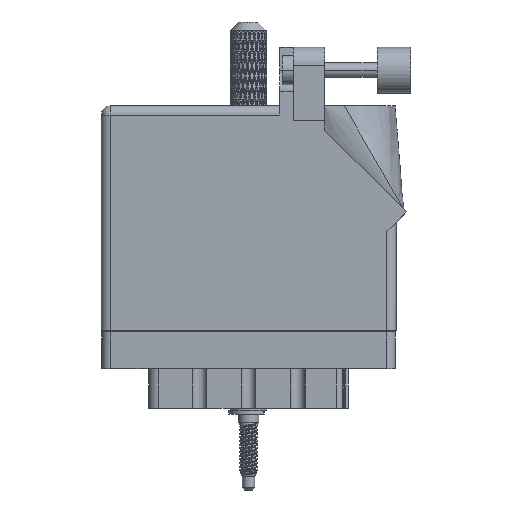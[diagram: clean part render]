
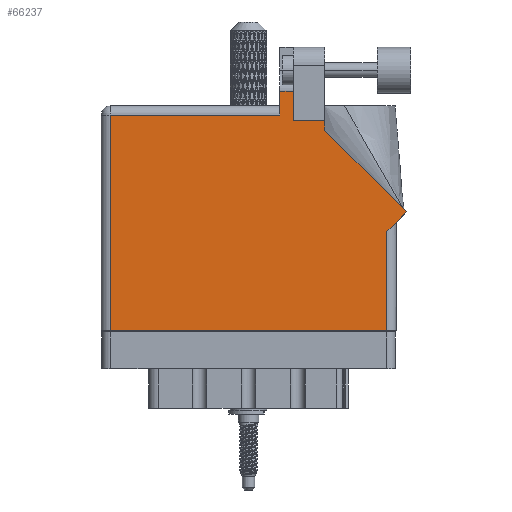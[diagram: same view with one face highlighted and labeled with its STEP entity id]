
A CAD part, front view. The second image highlights one B-rep face of the part: STEP entity #66237.
In plain terms, the highlighted face is planar.
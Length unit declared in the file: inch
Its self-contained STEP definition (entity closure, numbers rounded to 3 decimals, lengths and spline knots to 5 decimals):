
#945 = DIRECTION ( 'NONE',  ( -0.707, 0.707, 0. ) ) ;
#2197 = CARTESIAN_POINT ( 'NONE',  ( 1.948, 0.675, 0. ) ) ;
#3946 = LINE ( 'NONE', #8316, #59526 ) ;
#4428 = EDGE_CURVE ( 'NONE', #45870, #39399, #88461, .T. ) ;
#5207 = DIRECTION ( 'NONE',  ( -1., 0., 0. ) ) ;
#6542 = CARTESIAN_POINT ( 'NONE',  ( 2.01, 0.737, 0. ) ) ;
#7437 = VERTEX_POINT ( 'NONE', #2197 ) ;
#8316 = CARTESIAN_POINT ( 'NONE',  ( 1.948, 0.737, 0. ) ) ;
#9744 = VECTOR ( 'NONE', #44706, 39.37008 ) ;
#10318 = EDGE_CURVE ( 'NONE', #11266, #7437, #3946, .T. ) ;
#11266 = VERTEX_POINT ( 'NONE', #23895 ) ;
#11604 = EDGE_CURVE ( 'NONE', #39399, #94122, #60711, .T. ) ;
#12820 = CARTESIAN_POINT ( 'NONE',  ( 0., 0., 0. ) ) ;
#14624 = VECTOR ( 'NONE', #98952, 39.37008 ) ;
#14797 = VERTEX_POINT ( 'NONE', #15915 ) ;
#15915 = CARTESIAN_POINT ( 'NONE',  ( 0.062, 0., 0. ) ) ;
#16366 = LINE ( 'NONE', #43830, #66773 ) ;
#17846 = CARTESIAN_POINT ( 'NONE',  ( 1.311, 1.43, 0. ) ) ;
#18287 = VECTOR ( 'NONE', #106554, 39.37008 ) ;
#22402 = VECTOR ( 'NONE', #5207, 39.37008 ) ;
#23603 = LINE ( 'NONE', #41908, #72789 ) ;
#23895 = CARTESIAN_POINT ( 'NONE',  ( 1.948, 0., 0. ) ) ;
#25818 = VERTEX_POINT ( 'NONE', #58599 ) ;
#26074 = CARTESIAN_POINT ( 'NONE',  ( 1.311, 1.43, 0. ) ) ;
#26633 = CARTESIAN_POINT ( 'NONE',  ( 0., 1.53, 0. ) ) ;
#27106 = VECTOR ( 'NONE', #99921, 39.37008 ) ;
#27703 = DIRECTION ( 'NONE',  ( 0., 0., -1. ) ) ;
#27944 = CARTESIAN_POINT ( 'NONE',  ( 1.524, 1.36442, 0. ) ) ;
#29143 = CARTESIAN_POINT ( 'NONE',  ( 1.217, 1.6315, 0. ) ) ;
#31162 = ORIENTED_EDGE ( 'NONE', *, *, #10318, .T. ) ;
#33299 = DIRECTION ( 'NONE',  ( 0., 1., 0. ) ) ;
#36428 = VERTEX_POINT ( 'NONE', #27944 ) ;
#36837 = CARTESIAN_POINT ( 'NONE',  ( 1.524, 1.36442, 0. ) ) ;
#37196 = DIRECTION ( 'NONE',  ( 0., -1., 0. ) ) ;
#37208 = DIRECTION ( 'NONE',  ( 0., 1., 0. ) ) ;
#39399 = VERTEX_POINT ( 'NONE', #17846 ) ;
#39416 = VERTEX_POINT ( 'NONE', #102205 ) ;
#40521 = ORIENTED_EDGE ( 'NONE', *, *, #56850, .T. ) ;
#41908 = CARTESIAN_POINT ( 'NONE',  ( 2.08071, 0.80771, 0. ) ) ;
#43830 = CARTESIAN_POINT ( 'NONE',  ( 1.64177, 1.6315, 0. ) ) ;
#44706 = DIRECTION ( 'NONE',  ( 1., 0., 0. ) ) ;
#45870 = VERTEX_POINT ( 'NONE', #103061 ) ;
#48667 = CARTESIAN_POINT ( 'NONE',  ( 1.217, 1.53, 0. ) ) ;
#51704 = DIRECTION ( 'NONE',  ( 0.707, 0.707, 0. ) ) ;
#52444 = VECTOR ( 'NONE', #51704, 39.37008 ) ;
#56850 = EDGE_CURVE ( 'NONE', #81575, #36428, #23603, .T. ) ;
#57078 = EDGE_CURVE ( 'NONE', #90337, #39416, #67438, .T. ) ;
#58500 = ORIENTED_EDGE ( 'NONE', *, *, #78003, .T. ) ;
#58599 = CARTESIAN_POINT ( 'NONE',  ( 0.062, 1.468, 0. ) ) ;
#59398 = ORIENTED_EDGE ( 'NONE', *, *, #80004, .T. ) ;
#59526 = VECTOR ( 'NONE', #33299, 39.37008 ) ;
#60478 = ORIENTED_EDGE ( 'NONE', *, *, #4428, .T. ) ;
#60711 = LINE ( 'NONE', #26074, #27106 ) ;
#63185 = ORIENTED_EDGE ( 'NONE', *, *, #66318, .T. ) ;
#63223 = CARTESIAN_POINT ( 'NONE',  ( 2.08071, 0.80771, 0. ) ) ;
#63607 = ORIENTED_EDGE ( 'NONE', *, *, #57078, .T. ) ;
#65118 = EDGE_CURVE ( 'NONE', #94122, #90337, #16366, .T. ) ;
#66237 = ADVANCED_FACE ( 'NONE', ( #66673 ), #92501, .F. ) ;
#66318 = EDGE_CURVE ( 'NONE', #14797, #11266, #78350, .T. ) ;
#66673 = FACE_OUTER_BOUND ( 'NONE', #106581, .T. ) ;
#66773 = VECTOR ( 'NONE', #77066, 39.37008 ) ;
#67438 = LINE ( 'NONE', #48667, #18287 ) ;
#72789 = VECTOR ( 'NONE', #945, 39.37008 ) ;
#72917 = LINE ( 'NONE', #96103, #22402 ) ;
#74424 = LINE ( 'NONE', #36837, #106863 ) ;
#76862 = ORIENTED_EDGE ( 'NONE', *, *, #87516, .T. ) ;
#77066 = DIRECTION ( 'NONE',  ( -1., 0., 0. ) ) ;
#78003 = EDGE_CURVE ( 'NONE', #7437, #81575, #101712, .T. ) ;
#78350 = LINE ( 'NONE', #12820, #9744 ) ;
#78574 = CARTESIAN_POINT ( 'NONE',  ( 1.311, 1.6315, 0. ) ) ;
#78731 = CARTESIAN_POINT ( 'NONE',  ( 0.062, 0., 0. ) ) ;
#78922 = VECTOR ( 'NONE', #37196, 39.37008 ) ;
#80004 = EDGE_CURVE ( 'NONE', #39416, #25818, #72917, .T. ) ;
#81516 = CARTESIAN_POINT ( 'NONE',  ( 1.524, 1.43, 0. ) ) ;
#81575 = VERTEX_POINT ( 'NONE', #63223 ) ;
#85565 = DIRECTION ( 'NONE',  ( -1., 0., 0. ) ) ;
#87516 = EDGE_CURVE ( 'NONE', #36428, #45870, #74424, .T. ) ;
#88461 = LINE ( 'NONE', #81516, #14624 ) ;
#90337 = VERTEX_POINT ( 'NONE', #29143 ) ;
#90347 = AXIS2_PLACEMENT_3D ( 'NONE', #26633, #27703, #85565 ) ;
#92501 = PLANE ( 'NONE',  #90347 ) ;
#93832 = ORIENTED_EDGE ( 'NONE', *, *, #100796, .T. ) ;
#94122 = VERTEX_POINT ( 'NONE', #78574 ) ;
#96103 = CARTESIAN_POINT ( 'NONE',  ( 0., 1.468, 0. ) ) ;
#97158 = LINE ( 'NONE', #78731, #78922 ) ;
#98952 = DIRECTION ( 'NONE',  ( -1., 0., 0. ) ) ;
#99921 = DIRECTION ( 'NONE',  ( 0., 1., 0. ) ) ;
#100796 = EDGE_CURVE ( 'NONE', #25818, #14797, #97158, .T. ) ;
#101712 = LINE ( 'NONE', #6542, #52444 ) ;
#102205 = CARTESIAN_POINT ( 'NONE',  ( 1.217, 1.468, 0. ) ) ;
#103061 = CARTESIAN_POINT ( 'NONE',  ( 1.524, 1.43, 0. ) ) ;
#103521 = ORIENTED_EDGE ( 'NONE', *, *, #65118, .T. ) ;
#105424 = ORIENTED_EDGE ( 'NONE', *, *, #11604, .T. ) ;
#106554 = DIRECTION ( 'NONE',  ( 0., -1., 0. ) ) ;
#106581 = EDGE_LOOP ( 'NONE', ( #105424, #103521, #63607, #59398, #93832, #63185, #31162, #58500, #40521, #76862, #60478 ) ) ;
#106863 = VECTOR ( 'NONE', #37208, 39.37008 ) ;
